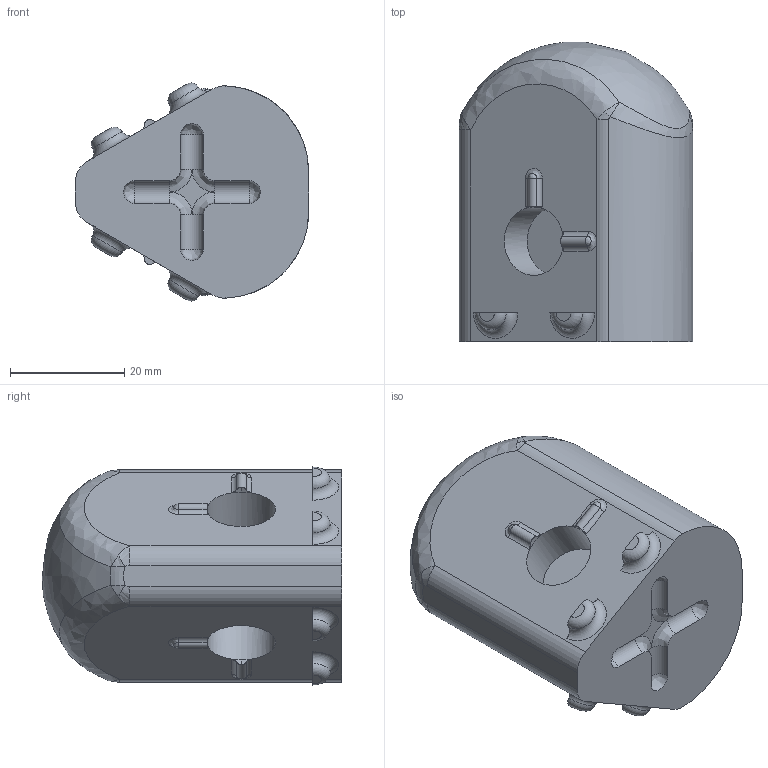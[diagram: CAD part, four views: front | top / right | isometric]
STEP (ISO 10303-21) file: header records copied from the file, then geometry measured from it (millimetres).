
FILE_DESCRIPTION (( 'STEP AP214' ), '1' );
FILE_NAME ('Short_Fore_Arm_V2.step', '2016-01-25T18:17:23', ( 'WarFairy' ), ( '' ), 'SwSTEP 2.0', 'SolidWorks 2015', '' );
FILE_SCHEMA (( 'AUTOMOTIVE_DESIGN' ));
Length unit declared in the file: inch
Products named in the file (1): Short_Fore_Arm_V2
Bounding box: 40.8 x 52.4 x 38.15 mm (x, y, z)
Volume: 48199.3 mm3; surface area: 8363.3 mm2
Topology: 1 solids, 1 shells, 101 faces, 248 edges, 148 vertices
Faces by surface type: bspline 53, cylinder 24, plane 16, torus 8
Full cylindrical faces by diameter (mm): 12 x2
Entity records: 4741 total; most frequent: CARTESIAN_POINT 2677, ORIENTED_EDGE 474, DIRECTION 362, EDGE_CURVE 237, AXIS2_PLACEMENT_3D 157, VERTEX_POINT 147, EDGE_LOOP 110, CIRCLE 108
